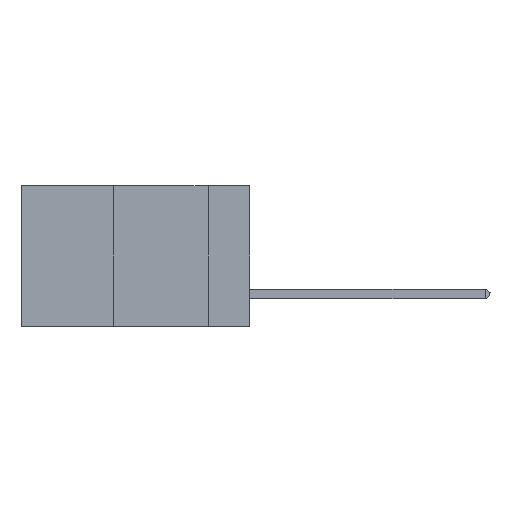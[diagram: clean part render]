
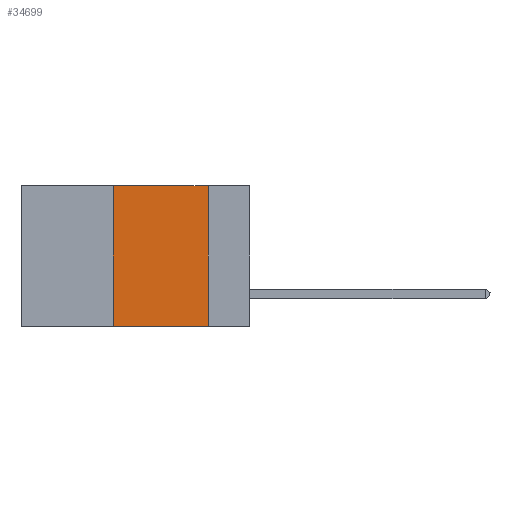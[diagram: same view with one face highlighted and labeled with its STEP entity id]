
A CAD part, left-side view. The second image highlights one B-rep face of the part: STEP entity #34699.
In plain terms, the highlighted planar face has unit normal (-1, 0, 0).
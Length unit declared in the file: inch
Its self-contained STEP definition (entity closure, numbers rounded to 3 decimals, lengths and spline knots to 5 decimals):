
#613 = LINE ( 'NONE', #3700, #37289 ) ;
#3548 = EDGE_LOOP ( 'NONE', ( #26415, #36180, #28890, #32024 ) ) ;
#3700 = CARTESIAN_POINT ( 'NONE',  ( 0., 0.36, 0. ) ) ;
#6495 = VERTEX_POINT ( 'NONE', #30559 ) ;
#6766 = CARTESIAN_POINT ( 'NONE',  ( 0., 0.11, -0.37 ) ) ;
#7103 = CARTESIAN_POINT ( 'NONE',  ( 0., 0.11, 0. ) ) ;
#8198 = EDGE_CURVE ( 'NONE', #25078, #32354, #25489, .T. ) ;
#11311 = LINE ( 'NONE', #7103, #34432 ) ;
#14062 = VERTEX_POINT ( 'NONE', #31268 ) ;
#14384 = PLANE ( 'NONE',  #16807 ) ;
#14650 = DIRECTION ( 'NONE',  ( 1., 0., 0. ) ) ;
#14793 = DIRECTION ( 'NONE',  ( 0., 0., -1. ) ) ;
#16807 = AXIS2_PLACEMENT_3D ( 'NONE', #36830, #14650, #14793 ) ;
#19974 = EDGE_CURVE ( 'NONE', #25078, #14062, #613, .T. ) ;
#20928 = VECTOR ( 'NONE', #23770, 39.37008 ) ;
#22678 = EDGE_CURVE ( 'NONE', #14062, #6495, #39110, .T. ) ;
#23770 = DIRECTION ( 'NONE',  ( 0., -1., 0. ) ) ;
#25078 = VERTEX_POINT ( 'NONE', #26918 ) ;
#25489 = LINE ( 'NONE', #39752, #20928 ) ;
#25601 = FACE_OUTER_BOUND ( 'NONE', #3548, .T. ) ;
#26415 = ORIENTED_EDGE ( 'NONE', *, *, #35772, .F. ) ;
#26918 = CARTESIAN_POINT ( 'NONE',  ( 0., 0.36, -0.37 ) ) ;
#28890 = ORIENTED_EDGE ( 'NONE', *, *, #19974, .F. ) ;
#29393 = DIRECTION ( 'NONE',  ( 0., 0., 1. ) ) ;
#29714 = DIRECTION ( 'NONE',  ( 0., 0., -1. ) ) ;
#30559 = CARTESIAN_POINT ( 'NONE',  ( 0., 0.11, 0. ) ) ;
#31268 = CARTESIAN_POINT ( 'NONE',  ( 0., 0.36, 0. ) ) ;
#31489 = CARTESIAN_POINT ( 'NONE',  ( 0., 0.6, 0. ) ) ;
#32024 = ORIENTED_EDGE ( 'NONE', *, *, #8198, .T. ) ;
#32354 = VERTEX_POINT ( 'NONE', #6766 ) ;
#34280 = DIRECTION ( 'NONE',  ( 0., -1., 0. ) ) ;
#34432 = VECTOR ( 'NONE', #29714, 39.37008 ) ;
#34699 = ADVANCED_FACE ( 'NONE', ( #25601 ), #14384, .F. ) ;
#35772 = EDGE_CURVE ( 'NONE', #6495, #32354, #11311, .T. ) ;
#36180 = ORIENTED_EDGE ( 'NONE', *, *, #22678, .F. ) ;
#36830 = CARTESIAN_POINT ( 'NONE',  ( 0., 0.6, 0. ) ) ;
#37289 = VECTOR ( 'NONE', #29393, 39.37008 ) ;
#39110 = LINE ( 'NONE', #31489, #40654 ) ;
#39752 = CARTESIAN_POINT ( 'NONE',  ( 0., 0.6, -0.37 ) ) ;
#40654 = VECTOR ( 'NONE', #34280, 39.37008 ) ;
